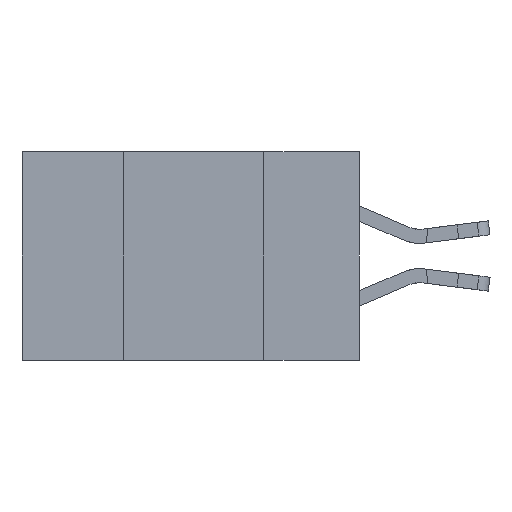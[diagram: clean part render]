
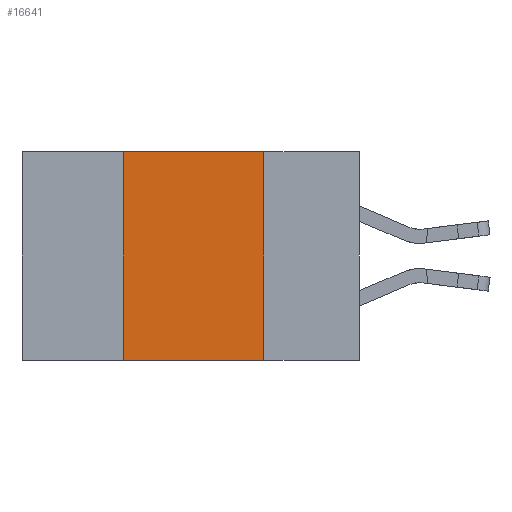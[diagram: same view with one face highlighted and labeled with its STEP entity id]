
A CAD part, left-side view. The second image highlights one B-rep face of the part: STEP entity #16641.
In plain terms, the highlighted planar face has unit normal (-1, 0, 0).
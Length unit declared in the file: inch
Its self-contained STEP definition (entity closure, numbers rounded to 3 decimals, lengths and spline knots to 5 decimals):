
#70 = DIRECTION ( 'NONE',  ( 0., 0., 1. ) ) ;
#633 = VECTOR ( 'NONE', #70, 39.37008 ) ;
#1142 = CARTESIAN_POINT ( 'NONE',  ( 0., 0.42, -0.37 ) ) ;
#1738 = FACE_OUTER_BOUND ( 'NONE', #6683, .T. ) ;
#2395 = VERTEX_POINT ( 'NONE', #10721 ) ;
#2577 = AXIS2_PLACEMENT_3D ( 'NONE', #5341, #12166, #14979 ) ;
#2610 = ORIENTED_EDGE ( 'NONE', *, *, #6561, .F. ) ;
#2974 = LINE ( 'NONE', #9797, #7328 ) ;
#4116 = ORIENTED_EDGE ( 'NONE', *, *, #10487, .F. ) ;
#4324 = PLANE ( 'NONE',  #2577 ) ;
#5341 = CARTESIAN_POINT ( 'NONE',  ( 0., 0.6, 0. ) ) ;
#5987 = EDGE_CURVE ( 'NONE', #2395, #14099, #17198, .T. ) ;
#6561 = EDGE_CURVE ( 'NONE', #14099, #10543, #2974, .T. ) ;
#6683 = EDGE_LOOP ( 'NONE', ( #2610, #11558, #4116, #12983 ) ) ;
#6774 = DIRECTION ( 'NONE',  ( 0., -1., 0. ) ) ;
#7151 = LINE ( 'NONE', #12385, #633 ) ;
#7328 = VECTOR ( 'NONE', #8529, 39.37008 ) ;
#7909 = VERTEX_POINT ( 'NONE', #1142 ) ;
#8386 = CARTESIAN_POINT ( 'NONE',  ( 0., 0.17, 0. ) ) ;
#8529 = DIRECTION ( 'NONE',  ( 0., 0., -1. ) ) ;
#8982 = CARTESIAN_POINT ( 'NONE',  ( 0., 0.6, -0.37 ) ) ;
#9401 = DIRECTION ( 'NONE',  ( 0., -1., 0. ) ) ;
#9797 = CARTESIAN_POINT ( 'NONE',  ( 0., 0.17, 0. ) ) ;
#10487 = EDGE_CURVE ( 'NONE', #7909, #2395, #7151, .T. ) ;
#10543 = VERTEX_POINT ( 'NONE', #16399 ) ;
#10721 = CARTESIAN_POINT ( 'NONE',  ( 0., 0.42, 0. ) ) ;
#11173 = VECTOR ( 'NONE', #6774, 39.37008 ) ;
#11558 = ORIENTED_EDGE ( 'NONE', *, *, #5987, .F. ) ;
#11867 = EDGE_CURVE ( 'NONE', #7909, #10543, #13063, .T. ) ;
#12166 = DIRECTION ( 'NONE',  ( 1., 0., 0. ) ) ;
#12385 = CARTESIAN_POINT ( 'NONE',  ( 0., 0.42, 0. ) ) ;
#12983 = ORIENTED_EDGE ( 'NONE', *, *, #11867, .T. ) ;
#13063 = LINE ( 'NONE', #8982, #14991 ) ;
#13568 = CARTESIAN_POINT ( 'NONE',  ( 0., 0.6, 0. ) ) ;
#14099 = VERTEX_POINT ( 'NONE', #8386 ) ;
#14979 = DIRECTION ( 'NONE',  ( 0., 0., -1. ) ) ;
#14991 = VECTOR ( 'NONE', #9401, 39.37008 ) ;
#16399 = CARTESIAN_POINT ( 'NONE',  ( 0., 0.17, -0.37 ) ) ;
#16641 = ADVANCED_FACE ( 'NONE', ( #1738 ), #4324, .F. ) ;
#17198 = LINE ( 'NONE', #13568, #11173 ) ;
